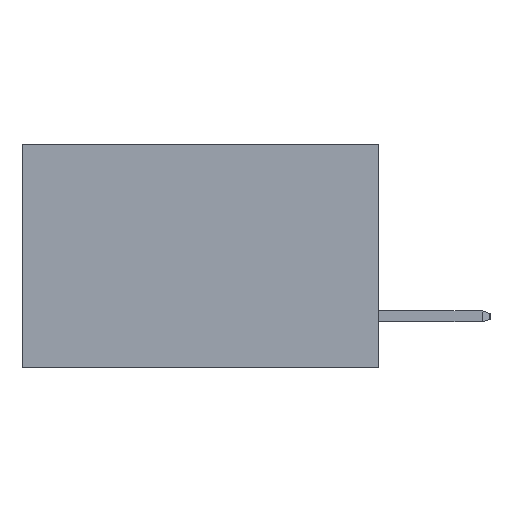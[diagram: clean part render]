
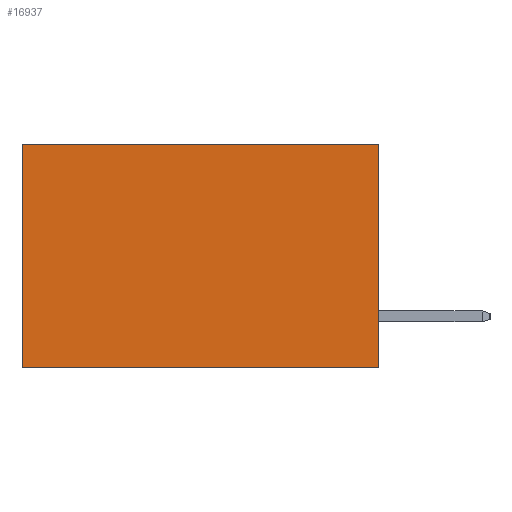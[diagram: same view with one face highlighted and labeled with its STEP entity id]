
A CAD part, left-side view. The second image highlights one B-rep face of the part: STEP entity #16937.
In plain terms, the highlighted planar face has unit normal (-1, 0, 0).
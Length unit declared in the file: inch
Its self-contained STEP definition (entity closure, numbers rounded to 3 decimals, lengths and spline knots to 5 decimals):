
#248 = CARTESIAN_POINT ( 'NONE',  ( 0.277, 0.59, -0.37 ) ) ;
#844 = FACE_OUTER_BOUND ( 'NONE', #8977, .T. ) ;
#1410 = DIRECTION ( 'NONE',  ( 0., 0., -1. ) ) ;
#1512 = LINE ( 'NONE', #248, #22552 ) ;
#1606 = DIRECTION ( 'NONE',  ( 0., 1., 0. ) ) ;
#2209 = VECTOR ( 'NONE', #12792, 39.37008 ) ;
#3395 = ORIENTED_EDGE ( 'NONE', *, *, #16507, .T. ) ;
#3749 = EDGE_CURVE ( 'NONE', #4670, #10931, #1512, .T. ) ;
#4575 = CARTESIAN_POINT ( 'NONE',  ( 0.277, 0., -0.37 ) ) ;
#4670 = VERTEX_POINT ( 'NONE', #20841 ) ;
#5080 = ORIENTED_EDGE ( 'NONE', *, *, #19222, .F. ) ;
#5198 = ORIENTED_EDGE ( 'NONE', *, *, #8044, .F. ) ;
#5383 = ORIENTED_EDGE ( 'NONE', *, *, #3749, .T. ) ;
#6299 = VECTOR ( 'NONE', #19990, 39.37008 ) ;
#7446 = LINE ( 'NONE', #12827, #2209 ) ;
#8044 = EDGE_CURVE ( 'NONE', #12770, #10931, #7446, .T. ) ;
#8090 = CARTESIAN_POINT ( 'NONE',  ( 0.277, 0., 0. ) ) ;
#8977 = EDGE_LOOP ( 'NONE', ( #5383, #5198, #5080, #3395 ) ) ;
#9154 = PLANE ( 'NONE',  #20813 ) ;
#10931 = VERTEX_POINT ( 'NONE', #12669 ) ;
#11083 = DIRECTION ( 'NONE',  ( 1., 0., 0. ) ) ;
#11441 = LINE ( 'NONE', #18115, #6299 ) ;
#12669 = CARTESIAN_POINT ( 'NONE',  ( 0.277, 0.59, -0.37 ) ) ;
#12770 = VERTEX_POINT ( 'NONE', #4575 ) ;
#12792 = DIRECTION ( 'NONE',  ( 0., 1., 0. ) ) ;
#12827 = CARTESIAN_POINT ( 'NONE',  ( 0.277, 0., -0.37 ) ) ;
#16507 = EDGE_CURVE ( 'NONE', #22548, #4670, #21359, .T. ) ;
#16937 = ADVANCED_FACE ( 'NONE', ( #844 ), #9154, .F. ) ;
#18115 = CARTESIAN_POINT ( 'NONE',  ( 0.277, 0., -0.37 ) ) ;
#19222 = EDGE_CURVE ( 'NONE', #22548, #12770, #11441, .T. ) ;
#19990 = DIRECTION ( 'NONE',  ( 0., 0., -1. ) ) ;
#20755 = VECTOR ( 'NONE', #1606, 39.37008 ) ;
#20813 = AXIS2_PLACEMENT_3D ( 'NONE', #22418, #11083, #24283 ) ;
#20841 = CARTESIAN_POINT ( 'NONE',  ( 0.277, 0.59, 0. ) ) ;
#21359 = LINE ( 'NONE', #24555, #20755 ) ;
#22418 = CARTESIAN_POINT ( 'NONE',  ( 0.277, 0., -0.37 ) ) ;
#22548 = VERTEX_POINT ( 'NONE', #8090 ) ;
#22552 = VECTOR ( 'NONE', #1410, 39.37008 ) ;
#24283 = DIRECTION ( 'NONE',  ( 0., 0., -1. ) ) ;
#24555 = CARTESIAN_POINT ( 'NONE',  ( 0.277, 0., 0. ) ) ;
